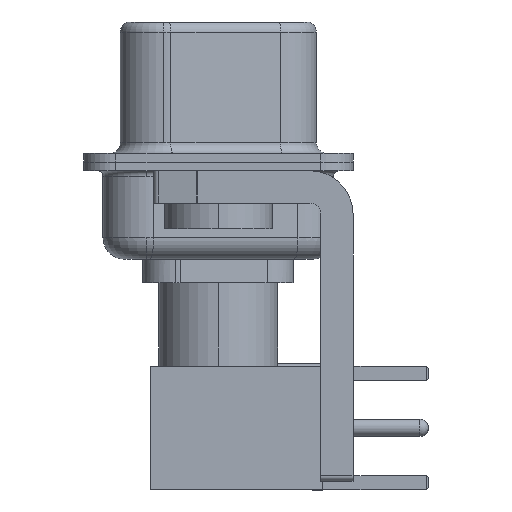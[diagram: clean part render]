
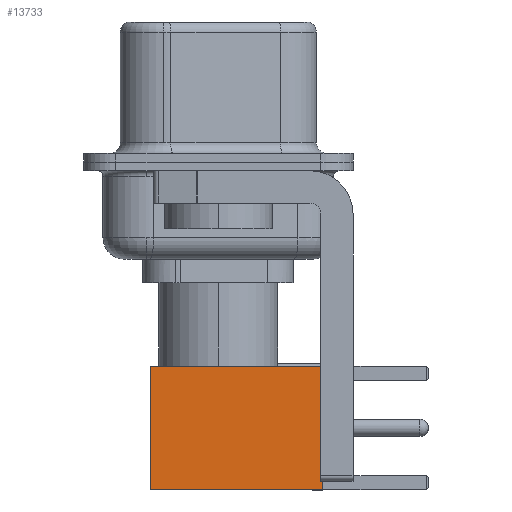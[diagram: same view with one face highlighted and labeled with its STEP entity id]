
A CAD part, left-side view. The second image highlights one B-rep face of the part: STEP entity #13733.
In plain terms, the highlighted face is planar.
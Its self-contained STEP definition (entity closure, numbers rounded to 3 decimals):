
#999 = DIRECTION ( 'NONE',  ( 0., 0., -1. ) ) ;
#1503 = DIRECTION ( 'NONE',  ( 0., 0., -1. ) ) ;
#1691 = VECTOR ( 'NONE', #18737, 1000. ) ;
#3029 = CARTESIAN_POINT ( 'NONE',  ( -2.875, 2.875, 8. ) ) ;
#3232 = VERTEX_POINT ( 'NONE', #14210 ) ;
#3484 = AXIS2_PLACEMENT_3D ( 'NONE', #26063, #11654, #19709 ) ;
#3682 = CARTESIAN_POINT ( 'NONE',  ( 2.875, 2.875, 8. ) ) ;
#3951 = ORIENTED_EDGE ( 'NONE', *, *, #20550, .F. ) ;
#5560 = FACE_OUTER_BOUND ( 'NONE', #9994, .T. ) ;
#5576 = VERTEX_POINT ( 'NONE', #19111 ) ;
#9024 = DIRECTION ( 'NONE',  ( -1., 0., 0. ) ) ;
#9994 = EDGE_LOOP ( 'NONE', ( #25899, #23934, #21449, #3951 ) ) ;
#10977 = EDGE_CURVE ( 'NONE', #5576, #3232, #17141, .T. ) ;
#11139 = CARTESIAN_POINT ( 'NONE',  ( 0., 2.875, 8. ) ) ;
#11654 = DIRECTION ( 'NONE',  ( 0., 1., 0. ) ) ;
#13106 = LINE ( 'NONE', #11139, #13410 ) ;
#13303 = LINE ( 'NONE', #25472, #17321 ) ;
#13410 = VECTOR ( 'NONE', #9024, 1000. ) ;
#13733 = ADVANCED_FACE ( 'NONE', ( #5560 ), #21707, .T. ) ;
#14210 = CARTESIAN_POINT ( 'NONE',  ( -2.875, 2.875, 0. ) ) ;
#17141 = LINE ( 'NONE', #24937, #1691 ) ;
#17321 = VECTOR ( 'NONE', #1503, 1000. ) ;
#18227 = VECTOR ( 'NONE', #999, 1000. ) ;
#18737 = DIRECTION ( 'NONE',  ( -1., 0., 0. ) ) ;
#19111 = CARTESIAN_POINT ( 'NONE',  ( 2.875, 2.875, 0. ) ) ;
#19268 = LINE ( 'NONE', #24964, #18227 ) ;
#19709 = DIRECTION ( 'NONE',  ( 0., 0., 1. ) ) ;
#20550 = EDGE_CURVE ( 'NONE', #21614, #25229, #13106, .T. ) ;
#21449 = ORIENTED_EDGE ( 'NONE', *, *, #24281, .F. ) ;
#21614 = VERTEX_POINT ( 'NONE', #3682 ) ;
#21707 = PLANE ( 'NONE',  #3484 ) ;
#23934 = ORIENTED_EDGE ( 'NONE', *, *, #10977, .T. ) ;
#24281 = EDGE_CURVE ( 'NONE', #25229, #3232, #13303, .T. ) ;
#24937 = CARTESIAN_POINT ( 'NONE',  ( 0., 2.875, 0. ) ) ;
#24964 = CARTESIAN_POINT ( 'NONE',  ( 2.875, 2.875, 0. ) ) ;
#25229 = VERTEX_POINT ( 'NONE', #3029 ) ;
#25472 = CARTESIAN_POINT ( 'NONE',  ( -2.875, 2.875, 0. ) ) ;
#25605 = EDGE_CURVE ( 'NONE', #21614, #5576, #19268, .T. ) ;
#25899 = ORIENTED_EDGE ( 'NONE', *, *, #25605, .T. ) ;
#26063 = CARTESIAN_POINT ( 'NONE',  ( 2.875, 2.875, 0. ) ) ;
